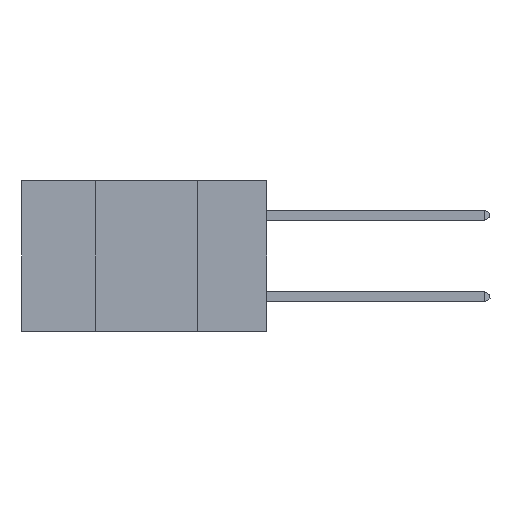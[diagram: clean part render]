
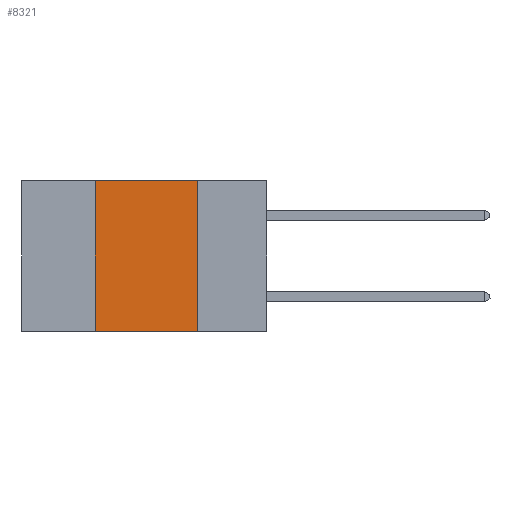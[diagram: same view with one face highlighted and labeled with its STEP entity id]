
A CAD part, left-side view. The second image highlights one B-rep face of the part: STEP entity #8321.
In plain terms, the highlighted planar face has unit normal (-1, 0, 0).
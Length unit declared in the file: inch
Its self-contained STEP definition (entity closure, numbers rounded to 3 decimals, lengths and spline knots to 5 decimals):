
#167 = VERTEX_POINT ( 'NONE', #16285 ) ;
#248 = VERTEX_POINT ( 'NONE', #446 ) ;
#270 = EDGE_CURVE ( 'NONE', #542, #248, #14603, .T. ) ;
#446 = CARTESIAN_POINT ( 'NONE',  ( 0., 0.17, -0.37 ) ) ;
#519 = DIRECTION ( 'NONE',  ( 0., -1., 0. ) ) ;
#542 = VERTEX_POINT ( 'NONE', #18456 ) ;
#792 = ORIENTED_EDGE ( 'NONE', *, *, #2520, .F. ) ;
#1077 = VECTOR ( 'NONE', #11180, 39.37008 ) ;
#1779 = VERTEX_POINT ( 'NONE', #14698 ) ;
#2371 = VECTOR ( 'NONE', #7566, 39.37008 ) ;
#2520 = EDGE_CURVE ( 'NONE', #1779, #167, #5073, .T. ) ;
#2857 = VECTOR ( 'NONE', #519, 39.37008 ) ;
#4865 = CARTESIAN_POINT ( 'NONE',  ( 0., 0.6, 0. ) ) ;
#4969 = FACE_OUTER_BOUND ( 'NONE', #15806, .T. ) ;
#5017 = ORIENTED_EDGE ( 'NONE', *, *, #270, .T. ) ;
#5073 = LINE ( 'NONE', #6730, #1077 ) ;
#6299 = ORIENTED_EDGE ( 'NONE', *, *, #17679, .F. ) ;
#6334 = DIRECTION ( 'NONE',  ( 1., 0., 0. ) ) ;
#6730 = CARTESIAN_POINT ( 'NONE',  ( 0., 0.6, 0. ) ) ;
#7566 = DIRECTION ( 'NONE',  ( 0., 0., -1. ) ) ;
#8319 = VECTOR ( 'NONE', #11278, 39.37008 ) ;
#8321 = ADVANCED_FACE ( 'NONE', ( #4969 ), #13634, .F. ) ;
#11080 = AXIS2_PLACEMENT_3D ( 'NONE', #4865, #6334, #16695 ) ;
#11180 = DIRECTION ( 'NONE',  ( 0., -1., 0. ) ) ;
#11278 = DIRECTION ( 'NONE',  ( 0., 0., 1. ) ) ;
#12588 = CARTESIAN_POINT ( 'NONE',  ( 0., 0.42, 0. ) ) ;
#13620 = LINE ( 'NONE', #16447, #2371 ) ;
#13634 = PLANE ( 'NONE',  #11080 ) ;
#14603 = LINE ( 'NONE', #15544, #2857 ) ;
#14698 = CARTESIAN_POINT ( 'NONE',  ( 0., 0.42, 0. ) ) ;
#15544 = CARTESIAN_POINT ( 'NONE',  ( 0., 0.6, -0.37 ) ) ;
#15806 = EDGE_LOOP ( 'NONE', ( #6299, #792, #16681, #5017 ) ) ;
#16216 = LINE ( 'NONE', #12588, #8319 ) ;
#16285 = CARTESIAN_POINT ( 'NONE',  ( 0., 0.17, 0. ) ) ;
#16447 = CARTESIAN_POINT ( 'NONE',  ( 0., 0.17, 0. ) ) ;
#16681 = ORIENTED_EDGE ( 'NONE', *, *, #18673, .F. ) ;
#16695 = DIRECTION ( 'NONE',  ( 0., 0., -1. ) ) ;
#17679 = EDGE_CURVE ( 'NONE', #167, #248, #13620, .T. ) ;
#18456 = CARTESIAN_POINT ( 'NONE',  ( 0., 0.42, -0.37 ) ) ;
#18673 = EDGE_CURVE ( 'NONE', #542, #1779, #16216, .T. ) ;
